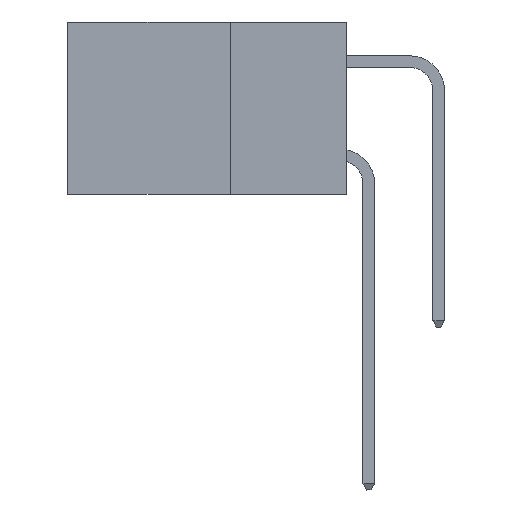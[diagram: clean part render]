
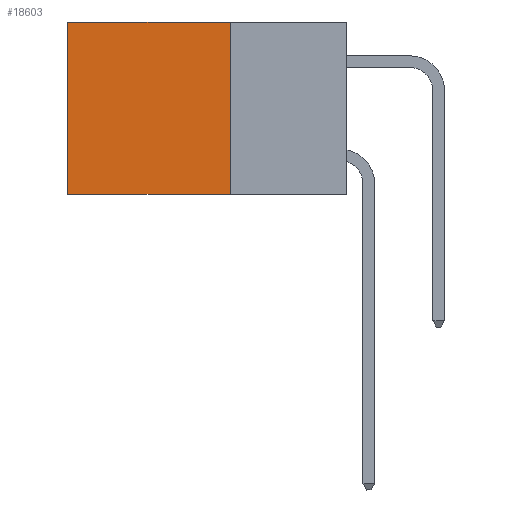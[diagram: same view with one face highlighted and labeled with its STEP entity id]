
A CAD part, left-side view. The second image highlights one B-rep face of the part: STEP entity #18603.
In plain terms, the highlighted planar face has unit normal (-1, 0, 0).
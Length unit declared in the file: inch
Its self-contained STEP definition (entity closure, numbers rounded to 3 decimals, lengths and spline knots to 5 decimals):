
#1769 = VERTEX_POINT ( 'NONE', #3605 ) ;
#2100 = CARTESIAN_POINT ( 'NONE',  ( 0.2875, 0.25, 0. ) ) ;
#2926 = ORIENTED_EDGE ( 'NONE', *, *, #20327, .F. ) ;
#3143 = DIRECTION ( 'NONE',  ( 0., 0., -1. ) ) ;
#3605 = CARTESIAN_POINT ( 'NONE',  ( 0.2875, 0.6, -0.37 ) ) ;
#3708 = DIRECTION ( 'NONE',  ( 0., 0., -1. ) ) ;
#4288 = CARTESIAN_POINT ( 'NONE',  ( 0.2875, 0.25, 0. ) ) ;
#4702 = VECTOR ( 'NONE', #20922, 39.37008 ) ;
#4785 = AXIS2_PLACEMENT_3D ( 'NONE', #28760, #28346, #3143 ) ;
#5618 = VERTEX_POINT ( 'NONE', #2100 ) ;
#7626 = LINE ( 'NONE', #14865, #24298 ) ;
#8715 = EDGE_CURVE ( 'NONE', #5618, #9658, #7626, .T. ) ;
#9238 = CARTESIAN_POINT ( 'NONE',  ( 0.2875, 0.6, 0. ) ) ;
#9658 = VERTEX_POINT ( 'NONE', #9238 ) ;
#9845 = PLANE ( 'NONE',  #4785 ) ;
#10717 = LINE ( 'NONE', #4288, #4702 ) ;
#10822 = LINE ( 'NONE', #17977, #21160 ) ;
#12236 = ORIENTED_EDGE ( 'NONE', *, *, #8715, .T. ) ;
#14865 = CARTESIAN_POINT ( 'NONE',  ( 0.2875, 0.25, 0. ) ) ;
#15091 = EDGE_LOOP ( 'NONE', ( #19070, #2926, #18158, #12236 ) ) ;
#15183 = DIRECTION ( 'NONE',  ( 0., 1., 0. ) ) ;
#16337 = DIRECTION ( 'NONE',  ( 0., 1., 0. ) ) ;
#17977 = CARTESIAN_POINT ( 'NONE',  ( 0.2875, 0.6, 0. ) ) ;
#18158 = ORIENTED_EDGE ( 'NONE', *, *, #19214, .F. ) ;
#18603 = ADVANCED_FACE ( 'NONE', ( #26674 ), #9845, .F. ) ;
#19070 = ORIENTED_EDGE ( 'NONE', *, *, #26525, .T. ) ;
#19214 = EDGE_CURVE ( 'NONE', #5618, #30110, #10717, .T. ) ;
#20327 = EDGE_CURVE ( 'NONE', #30110, #1769, #29514, .T. ) ;
#20922 = DIRECTION ( 'NONE',  ( 0., 0., -1. ) ) ;
#21160 = VECTOR ( 'NONE', #3708, 39.37008 ) ;
#23343 = CARTESIAN_POINT ( 'NONE',  ( 0.2875, 0.25, -0.37 ) ) ;
#24298 = VECTOR ( 'NONE', #15183, 39.37008 ) ;
#25035 = CARTESIAN_POINT ( 'NONE',  ( 0.2875, 0.25, -0.37 ) ) ;
#26200 = VECTOR ( 'NONE', #16337, 39.37008 ) ;
#26525 = EDGE_CURVE ( 'NONE', #9658, #1769, #10822, .T. ) ;
#26674 = FACE_OUTER_BOUND ( 'NONE', #15091, .T. ) ;
#28346 = DIRECTION ( 'NONE',  ( 1., 0., 0. ) ) ;
#28760 = CARTESIAN_POINT ( 'NONE',  ( 0.2875, 0.25, 0. ) ) ;
#29514 = LINE ( 'NONE', #23343, #26200 ) ;
#30110 = VERTEX_POINT ( 'NONE', #25035 ) ;
